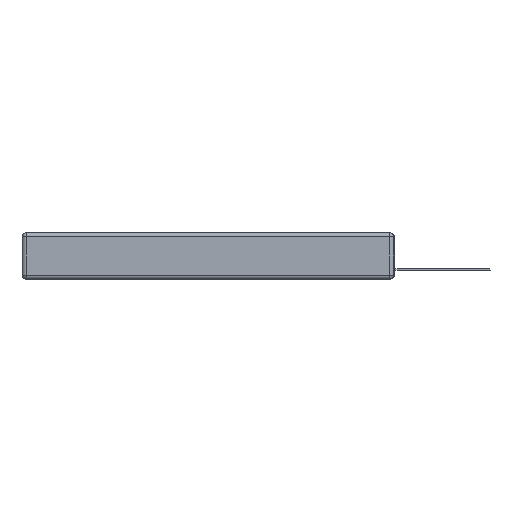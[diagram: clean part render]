
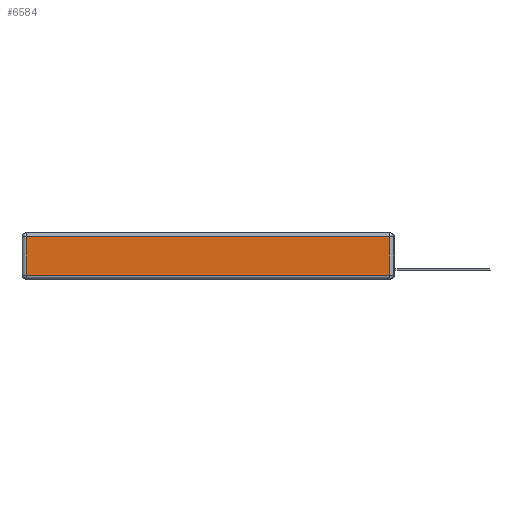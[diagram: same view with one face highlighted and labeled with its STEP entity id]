
A CAD part, left-side view. The second image highlights one B-rep face of the part: STEP entity #6584.
In plain terms, the highlighted planar face has unit normal (-1, 0, 0).
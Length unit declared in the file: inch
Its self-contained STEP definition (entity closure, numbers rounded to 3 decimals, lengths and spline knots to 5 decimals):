
#51 = CARTESIAN_POINT ( 'NONE',  ( 0., 0., -0.343 ) ) ;
#1580 = VECTOR ( 'NONE', #17198, 39.37008 ) ;
#2112 = VECTOR ( 'NONE', #6494, 39.37008 ) ;
#2736 = DIRECTION ( 'NONE',  ( -1., 0., 0. ) ) ;
#2829 = EDGE_CURVE ( 'NONE', #15846, #3755, #5132, .T. ) ;
#3524 = ORIENTED_EDGE ( 'NONE', *, *, #15341, .T. ) ;
#3755 = VERTEX_POINT ( 'NONE', #6532 ) ;
#4651 = CARTESIAN_POINT ( 'NONE',  ( 0., 0.03, -0.03 ) ) ;
#5132 = LINE ( 'NONE', #14515, #1580 ) ;
#5203 = PLANE ( 'NONE',  #10163 ) ;
#5296 = EDGE_LOOP ( 'NONE', ( #8575, #12828, #14160, #3524 ) ) ;
#6356 = DIRECTION ( 'NONE',  ( 0., 1., 0. ) ) ;
#6494 = DIRECTION ( 'NONE',  ( 0., 0., 1. ) ) ;
#6532 = CARTESIAN_POINT ( 'NONE',  ( 0., 0.03, -0.313 ) ) ;
#6584 = ADVANCED_FACE ( 'NONE', ( #16905 ), #5203, .T. ) ;
#6800 = DIRECTION ( 'NONE',  ( 0., 0., 1. ) ) ;
#7432 = EDGE_CURVE ( 'NONE', #3755, #9254, #13737, .T. ) ;
#8575 = ORIENTED_EDGE ( 'NONE', *, *, #2829, .T. ) ;
#8589 = LINE ( 'NONE', #12128, #8990 ) ;
#8990 = VECTOR ( 'NONE', #14876, 39.37008 ) ;
#9033 = CARTESIAN_POINT ( 'NONE',  ( 0., 0.03, -0.343 ) ) ;
#9254 = VERTEX_POINT ( 'NONE', #4651 ) ;
#10163 = AXIS2_PLACEMENT_3D ( 'NONE', #51, #2736, #6800 ) ;
#10427 = CARTESIAN_POINT ( 'NONE',  ( 0., 2.75, -0.03 ) ) ;
#11790 = VERTEX_POINT ( 'NONE', #12673 ) ;
#12128 = CARTESIAN_POINT ( 'NONE',  ( 0., 2.72, -0.343 ) ) ;
#12579 = LINE ( 'NONE', #10427, #15141 ) ;
#12673 = CARTESIAN_POINT ( 'NONE',  ( 0., 2.72, -0.03 ) ) ;
#12828 = ORIENTED_EDGE ( 'NONE', *, *, #7432, .T. ) ;
#13737 = LINE ( 'NONE', #9033, #2112 ) ;
#14160 = ORIENTED_EDGE ( 'NONE', *, *, #15177, .T. ) ;
#14515 = CARTESIAN_POINT ( 'NONE',  ( 0., 0., -0.313 ) ) ;
#14876 = DIRECTION ( 'NONE',  ( 0., 0., -1. ) ) ;
#15141 = VECTOR ( 'NONE', #6356, 39.37008 ) ;
#15177 = EDGE_CURVE ( 'NONE', #9254, #11790, #12579, .T. ) ;
#15341 = EDGE_CURVE ( 'NONE', #11790, #15846, #8589, .T. ) ;
#15846 = VERTEX_POINT ( 'NONE', #16003 ) ;
#16003 = CARTESIAN_POINT ( 'NONE',  ( 0., 2.72, -0.313 ) ) ;
#16905 = FACE_OUTER_BOUND ( 'NONE', #5296, .T. ) ;
#17198 = DIRECTION ( 'NONE',  ( 0., -1., 0. ) ) ;
